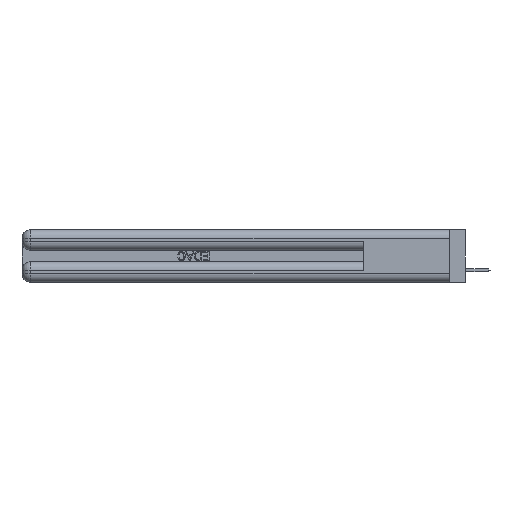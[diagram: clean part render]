
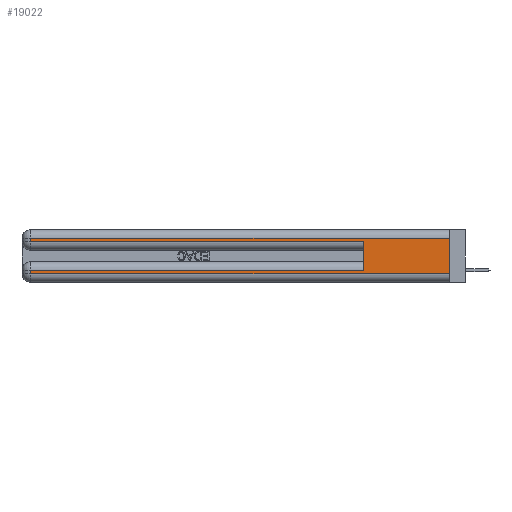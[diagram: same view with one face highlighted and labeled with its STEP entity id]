
A CAD part, left-side view. The second image highlights one B-rep face of the part: STEP entity #19022.
In plain terms, the highlighted planar face has unit normal (-1, 0, 0).
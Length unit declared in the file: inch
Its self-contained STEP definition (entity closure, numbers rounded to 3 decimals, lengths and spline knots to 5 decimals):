
#1002 = CARTESIAN_POINT ( 'NONE',  ( 0., 0., 0.31 ) ) ;
#5613 = ORIENTED_EDGE ( 'NONE', *, *, #46075, .T. ) ;
#5629 = DIRECTION ( 'NONE',  ( 0., -1., 0. ) ) ;
#6126 = LINE ( 'NONE', #40607, #8994 ) ;
#6995 = EDGE_CURVE ( 'NONE', #10591, #33308, #33208, .T. ) ;
#7282 = DIRECTION ( 'NONE',  ( 0., 0., -1. ) ) ;
#8994 = VECTOR ( 'NONE', #7282, 39.37008 ) ;
#9442 = VERTEX_POINT ( 'NONE', #20831 ) ;
#9624 = LINE ( 'NONE', #27938, #47978 ) ;
#9979 = EDGE_CURVE ( 'NONE', #9442, #27552, #6126, .T. ) ;
#10591 = VERTEX_POINT ( 'NONE', #17489 ) ;
#11133 = EDGE_LOOP ( 'NONE', ( #46753, #43259, #11973, #47429, #43143, #35318, #17954, #5613 ) ) ;
#11906 = CARTESIAN_POINT ( 'NONE',  ( 0., 2.94, 0.31 ) ) ;
#11973 = ORIENTED_EDGE ( 'NONE', *, *, #26134, .T. ) ;
#12459 = AXIS2_PLACEMENT_3D ( 'NONE', #27395, #38589, #45392 ) ;
#13175 = EDGE_CURVE ( 'NONE', #9442, #16480, #46464, .T. ) ;
#16480 = VERTEX_POINT ( 'NONE', #11906 ) ;
#16675 = CARTESIAN_POINT ( 'NONE',  ( 0., 0., 0.285 ) ) ;
#17125 = LINE ( 'NONE', #19704, #18821 ) ;
#17489 = CARTESIAN_POINT ( 'NONE',  ( 0., 2.94, 0.085 ) ) ;
#17954 = ORIENTED_EDGE ( 'NONE', *, *, #6995, .T. ) ;
#18727 = EDGE_CURVE ( 'NONE', #35047, #22277, #29399, .T. ) ;
#18821 = VECTOR ( 'NONE', #38237, 39.37008 ) ;
#19022 = ADVANCED_FACE ( 'NONE', ( #22895 ), #45725, .F. ) ;
#19432 = VECTOR ( 'NONE', #5629, 39.37008 ) ;
#19704 = CARTESIAN_POINT ( 'NONE',  ( 0., 0., 0.085 ) ) ;
#20425 = CARTESIAN_POINT ( 'NONE',  ( 0., 2.94, 0.37 ) ) ;
#20829 = CARTESIAN_POINT ( 'NONE',  ( 0., 2.94, 0.37 ) ) ;
#20831 = CARTESIAN_POINT ( 'NONE',  ( 0., 0., 0.31 ) ) ;
#22277 = VERTEX_POINT ( 'NONE', #31005 ) ;
#22895 = FACE_OUTER_BOUND ( 'NONE', #11133, .T. ) ;
#26134 = EDGE_CURVE ( 'NONE', #16480, #35047, #28347, .T. ) ;
#27395 = CARTESIAN_POINT ( 'NONE',  ( 0., 0., 0.37 ) ) ;
#27552 = VERTEX_POINT ( 'NONE', #36633 ) ;
#27938 = CARTESIAN_POINT ( 'NONE',  ( 0., 0., 0.06 ) ) ;
#28347 = LINE ( 'NONE', #20425, #37057 ) ;
#29399 = LINE ( 'NONE', #16675, #19432 ) ;
#29976 = DIRECTION ( 'NONE',  ( 0., 0., 1. ) ) ;
#30893 = DIRECTION ( 'NONE',  ( 0., 1., 0. ) ) ;
#31005 = CARTESIAN_POINT ( 'NONE',  ( 0., 0.6, 0.285 ) ) ;
#31850 = DIRECTION ( 'NONE',  ( 0., -1., 0. ) ) ;
#33059 = CARTESIAN_POINT ( 'NONE',  ( 0., 2.94, 0.06 ) ) ;
#33208 = LINE ( 'NONE', #20829, #34343 ) ;
#33308 = VERTEX_POINT ( 'NONE', #33059 ) ;
#33949 = EDGE_CURVE ( 'NONE', #45317, #22277, #40569, .T. ) ;
#34343 = VECTOR ( 'NONE', #40317, 39.37008 ) ;
#35047 = VERTEX_POINT ( 'NONE', #44038 ) ;
#35318 = ORIENTED_EDGE ( 'NONE', *, *, #35989, .T. ) ;
#35989 = EDGE_CURVE ( 'NONE', #45317, #10591, #17125, .T. ) ;
#36633 = CARTESIAN_POINT ( 'NONE',  ( 0., 0., 0.06 ) ) ;
#37057 = VECTOR ( 'NONE', #38801, 39.37008 ) ;
#38237 = DIRECTION ( 'NONE',  ( 0., 1., 0. ) ) ;
#38589 = DIRECTION ( 'NONE',  ( 1., 0., 0. ) ) ;
#38801 = DIRECTION ( 'NONE',  ( 0., 0., -1. ) ) ;
#40317 = DIRECTION ( 'NONE',  ( 0., 0., -1. ) ) ;
#40569 = LINE ( 'NONE', #45204, #45167 ) ;
#40607 = CARTESIAN_POINT ( 'NONE',  ( 0., 0., 0.37 ) ) ;
#43143 = ORIENTED_EDGE ( 'NONE', *, *, #33949, .F. ) ;
#43259 = ORIENTED_EDGE ( 'NONE', *, *, #13175, .T. ) ;
#44038 = CARTESIAN_POINT ( 'NONE',  ( 0., 2.94, 0.285 ) ) ;
#45167 = VECTOR ( 'NONE', #29976, 39.37008 ) ;
#45204 = CARTESIAN_POINT ( 'NONE',  ( 0., 0.6, 0.145 ) ) ;
#45317 = VERTEX_POINT ( 'NONE', #47747 ) ;
#45392 = DIRECTION ( 'NONE',  ( 0., 0., -1. ) ) ;
#45725 = PLANE ( 'NONE',  #12459 ) ;
#46075 = EDGE_CURVE ( 'NONE', #33308, #27552, #9624, .T. ) ;
#46464 = LINE ( 'NONE', #1002, #47669 ) ;
#46753 = ORIENTED_EDGE ( 'NONE', *, *, #9979, .F. ) ;
#47429 = ORIENTED_EDGE ( 'NONE', *, *, #18727, .T. ) ;
#47669 = VECTOR ( 'NONE', #30893, 39.37008 ) ;
#47747 = CARTESIAN_POINT ( 'NONE',  ( 0., 0.6, 0.085 ) ) ;
#47978 = VECTOR ( 'NONE', #31850, 39.37008 ) ;
